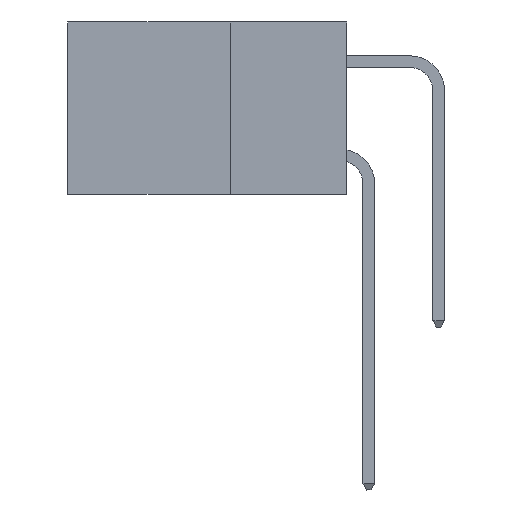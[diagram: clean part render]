
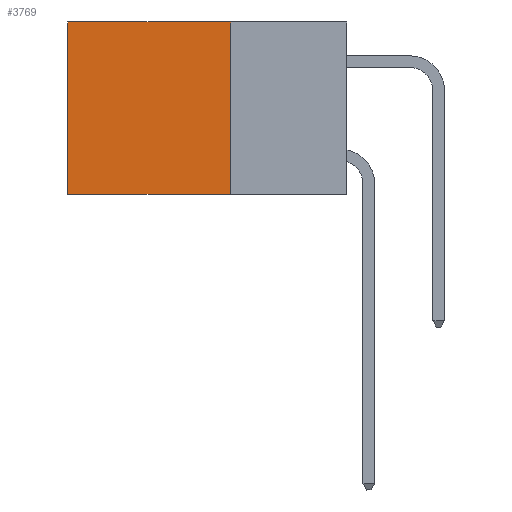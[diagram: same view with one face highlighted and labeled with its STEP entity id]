
A CAD part, left-side view. The second image highlights one B-rep face of the part: STEP entity #3769.
In plain terms, the highlighted planar face has unit normal (-1, 0, 0).
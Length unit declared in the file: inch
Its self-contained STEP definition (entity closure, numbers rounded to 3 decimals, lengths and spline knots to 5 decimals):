
#282 = CARTESIAN_POINT ( 'NONE',  ( 0.2875, 0.25, 0. ) ) ;
#352 = VECTOR ( 'NONE', #3794, 39.37008 ) ;
#411 = CARTESIAN_POINT ( 'NONE',  ( 0.2875, 0.6, 0. ) ) ;
#877 = ORIENTED_EDGE ( 'NONE', *, *, #11830, .F. ) ;
#1318 = CARTESIAN_POINT ( 'NONE',  ( 0.2875, 0.25, 0. ) ) ;
#2182 = ORIENTED_EDGE ( 'NONE', *, *, #10188, .F. ) ;
#2368 = DIRECTION ( 'NONE',  ( 0., 0., -1. ) ) ;
#2761 = LINE ( 'NONE', #11197, #11516 ) ;
#3128 = DIRECTION ( 'NONE',  ( 0., 1., 0. ) ) ;
#3769 = ADVANCED_FACE ( 'NONE', ( #13589 ), #3961, .F. ) ;
#3794 = DIRECTION ( 'NONE',  ( 0., 1., 0. ) ) ;
#3961 = PLANE ( 'NONE',  #4423 ) ;
#4423 = AXIS2_PLACEMENT_3D ( 'NONE', #9626, #11019, #15532 ) ;
#4861 = VERTEX_POINT ( 'NONE', #10259 ) ;
#5043 = ORIENTED_EDGE ( 'NONE', *, *, #10054, .T. ) ;
#5233 = VECTOR ( 'NONE', #3128, 39.37008 ) ;
#5271 = CARTESIAN_POINT ( 'NONE',  ( 0.2875, 0.25, -0.37 ) ) ;
#6164 = CARTESIAN_POINT ( 'NONE',  ( 0.2875, 0.25, 0. ) ) ;
#7013 = VERTEX_POINT ( 'NONE', #411 ) ;
#9333 = VECTOR ( 'NONE', #2368, 39.37008 ) ;
#9600 = VERTEX_POINT ( 'NONE', #6164 ) ;
#9626 = CARTESIAN_POINT ( 'NONE',  ( 0.2875, 0.25, 0. ) ) ;
#10054 = EDGE_CURVE ( 'NONE', #9600, #7013, #12559, .T. ) ;
#10188 = EDGE_CURVE ( 'NONE', #4861, #18471, #12089, .T. ) ;
#10259 = CARTESIAN_POINT ( 'NONE',  ( 0.2875, 0.25, -0.37 ) ) ;
#10964 = LINE ( 'NONE', #1318, #9333 ) ;
#11019 = DIRECTION ( 'NONE',  ( 1., 0., 0. ) ) ;
#11197 = CARTESIAN_POINT ( 'NONE',  ( 0.2875, 0.6, 0. ) ) ;
#11516 = VECTOR ( 'NONE', #15635, 39.37008 ) ;
#11830 = EDGE_CURVE ( 'NONE', #9600, #4861, #10964, .T. ) ;
#12089 = LINE ( 'NONE', #5271, #352 ) ;
#12559 = LINE ( 'NONE', #282, #5233 ) ;
#13589 = FACE_OUTER_BOUND ( 'NONE', #16914, .T. ) ;
#15282 = EDGE_CURVE ( 'NONE', #7013, #18471, #2761, .T. ) ;
#15532 = DIRECTION ( 'NONE',  ( 0., 0., -1. ) ) ;
#15635 = DIRECTION ( 'NONE',  ( 0., 0., -1. ) ) ;
#16914 = EDGE_LOOP ( 'NONE', ( #17465, #2182, #877, #5043 ) ) ;
#17465 = ORIENTED_EDGE ( 'NONE', *, *, #15282, .T. ) ;
#18471 = VERTEX_POINT ( 'NONE', #18755 ) ;
#18755 = CARTESIAN_POINT ( 'NONE',  ( 0.2875, 0.6, -0.37 ) ) ;
